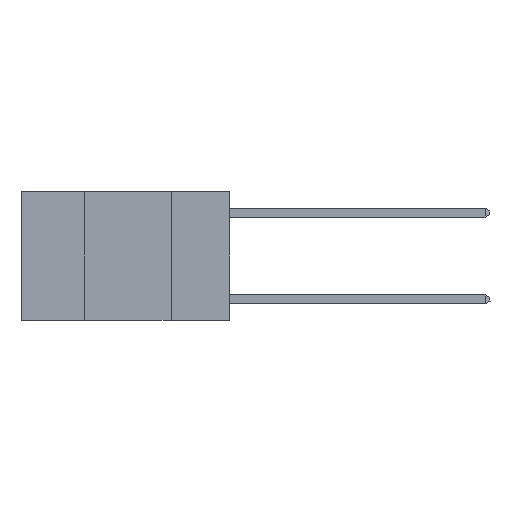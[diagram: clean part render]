
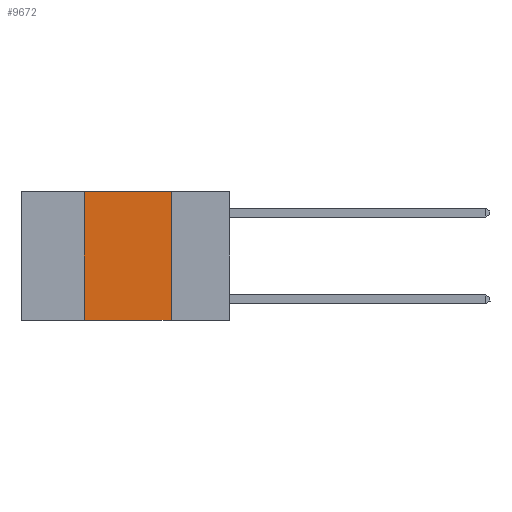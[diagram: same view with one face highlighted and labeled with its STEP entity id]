
A CAD part, left-side view. The second image highlights one B-rep face of the part: STEP entity #9672.
In plain terms, the highlighted planar face has unit normal (-1, 0, 0).
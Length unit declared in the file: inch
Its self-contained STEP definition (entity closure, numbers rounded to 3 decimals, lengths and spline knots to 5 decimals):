
#1099 = PLANE ( 'NONE',  #17426 ) ;
#2101 = CARTESIAN_POINT ( 'NONE',  ( 0., 0.6, -0.37 ) ) ;
#2164 = VERTEX_POINT ( 'NONE', #19237 ) ;
#2207 = VECTOR ( 'NONE', #5112, 39.37008 ) ;
#2771 = CARTESIAN_POINT ( 'NONE',  ( 0., 0.42, 0. ) ) ;
#3043 = CARTESIAN_POINT ( 'NONE',  ( 0., 0.42, -0.37 ) ) ;
#3188 = CARTESIAN_POINT ( 'NONE',  ( 0., 0.17, -0.37 ) ) ;
#3821 = ORIENTED_EDGE ( 'NONE', *, *, #25258, .F. ) ;
#4302 = EDGE_LOOP ( 'NONE', ( #14734, #3821, #16180, #4558 ) ) ;
#4558 = ORIENTED_EDGE ( 'NONE', *, *, #15241, .T. ) ;
#4807 = VECTOR ( 'NONE', #23308, 39.37008 ) ;
#5112 = DIRECTION ( 'NONE',  ( 0., 0., 1. ) ) ;
#5351 = LINE ( 'NONE', #17826, #29058 ) ;
#5799 = DIRECTION ( 'NONE',  ( 1., 0., 0. ) ) ;
#5954 = LINE ( 'NONE', #2101, #23611 ) ;
#6419 = FACE_OUTER_BOUND ( 'NONE', #4302, .T. ) ;
#8139 = VERTEX_POINT ( 'NONE', #15373 ) ;
#9672 = ADVANCED_FACE ( 'NONE', ( #6419 ), #1099, .F. ) ;
#10995 = LINE ( 'NONE', #21035, #4807 ) ;
#13701 = DIRECTION ( 'NONE',  ( 0., -1., 0. ) ) ;
#14734 = ORIENTED_EDGE ( 'NONE', *, *, #19883, .F. ) ;
#15241 = EDGE_CURVE ( 'NONE', #20935, #28253, #5954, .T. ) ;
#15373 = CARTESIAN_POINT ( 'NONE',  ( 0., 0.17, 0. ) ) ;
#16180 = ORIENTED_EDGE ( 'NONE', *, *, #16789, .F. ) ;
#16789 = EDGE_CURVE ( 'NONE', #20935, #2164, #20686, .T. ) ;
#17426 = AXIS2_PLACEMENT_3D ( 'NONE', #19680, #5799, #21922 ) ;
#17826 = CARTESIAN_POINT ( 'NONE',  ( 0., 0.17, 0. ) ) ;
#19237 = CARTESIAN_POINT ( 'NONE',  ( 0., 0.42, 0. ) ) ;
#19680 = CARTESIAN_POINT ( 'NONE',  ( 0., 0.6, 0. ) ) ;
#19883 = EDGE_CURVE ( 'NONE', #8139, #28253, #5351, .T. ) ;
#20686 = LINE ( 'NONE', #2771, #2207 ) ;
#20935 = VERTEX_POINT ( 'NONE', #3043 ) ;
#21035 = CARTESIAN_POINT ( 'NONE',  ( 0., 0.6, 0. ) ) ;
#21922 = DIRECTION ( 'NONE',  ( 0., 0., -1. ) ) ;
#23308 = DIRECTION ( 'NONE',  ( 0., -1., 0. ) ) ;
#23611 = VECTOR ( 'NONE', #13701, 39.37008 ) ;
#24675 = DIRECTION ( 'NONE',  ( 0., 0., -1. ) ) ;
#25258 = EDGE_CURVE ( 'NONE', #2164, #8139, #10995, .T. ) ;
#28253 = VERTEX_POINT ( 'NONE', #3188 ) ;
#29058 = VECTOR ( 'NONE', #24675, 39.37008 ) ;
